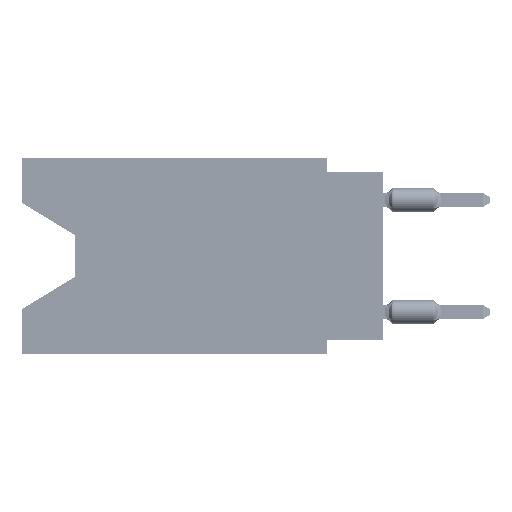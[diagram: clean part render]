
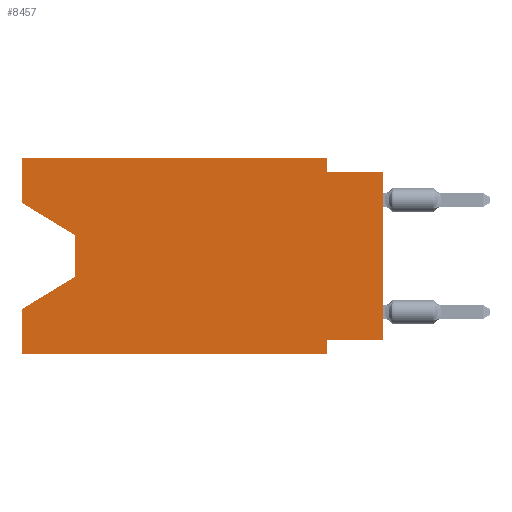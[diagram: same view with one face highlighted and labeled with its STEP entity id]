
A CAD part, left-side view. The second image highlights one B-rep face of the part: STEP entity #8457.
In plain terms, the highlighted planar face has unit normal (-1, 0, 0).
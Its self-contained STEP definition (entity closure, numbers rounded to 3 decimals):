
#1317 = ORIENTED_EDGE ( 'NONE', *, *, #39299, .T. ) ;
#1532 = DIRECTION ( 'NONE',  ( 0., -1., 0. ) ) ;
#1831 = EDGE_CURVE ( 'NONE', #32537, #29362, #54816, .T. ) ;
#2239 = DIRECTION ( 'NONE',  ( 0., 1., 0. ) ) ;
#2278 = LINE ( 'NONE', #7895, #40088 ) ;
#2956 = EDGE_CURVE ( 'NONE', #59551, #34029, #50661, .T. ) ;
#6579 = EDGE_CURVE ( 'NONE', #72040, #9391, #73332, .T. ) ;
#7839 = EDGE_CURVE ( 'NONE', #36415, #64569, #8809, .T. ) ;
#7856 = CARTESIAN_POINT ( 'NONE',  ( 0., 13.97, -3.505 ) ) ;
#7895 = CARTESIAN_POINT ( 'NONE',  ( 0., 0., -0.635 ) ) ;
#8457 = ADVANCED_FACE ( 'NONE', ( #12666 ), #17926, .F. ) ;
#8486 = VECTOR ( 'NONE', #14846, 1000. ) ;
#8809 = LINE ( 'NONE', #20768, #47941 ) ;
#9391 = VERTEX_POINT ( 'NONE', #51396 ) ;
#11251 = CARTESIAN_POINT ( 'NONE',  ( 0., 16.383, -8.89 ) ) ;
#12129 = EDGE_CURVE ( 'NONE', #32537, #13895, #23653, .T. ) ;
#12666 = FACE_OUTER_BOUND ( 'NONE', #43192, .T. ) ;
#13191 = VECTOR ( 'NONE', #67030, 1000. ) ;
#13895 = VERTEX_POINT ( 'NONE', #16146 ) ;
#14657 = CARTESIAN_POINT ( 'NONE',  ( 0., 2.54, 0. ) ) ;
#14846 = DIRECTION ( 'NONE',  ( 0., -1., 0. ) ) ;
#16146 = CARTESIAN_POINT ( 'NONE',  ( 0., 16.383, 0. ) ) ;
#17688 = CARTESIAN_POINT ( 'NONE',  ( 0., 16.383, -6.852 ) ) ;
#17926 = PLANE ( 'NONE',  #39604 ) ;
#19988 = LINE ( 'NONE', #38624, #63804 ) ;
#20069 = DIRECTION ( 'NONE',  ( 0., 0., -1. ) ) ;
#20768 = CARTESIAN_POINT ( 'NONE',  ( 0., 2.54, 0. ) ) ;
#22846 = ORIENTED_EDGE ( 'NONE', *, *, #31156, .F. ) ;
#23537 = CARTESIAN_POINT ( 'NONE',  ( 0., 16.383, 0. ) ) ;
#23653 = LINE ( 'NONE', #34512, #50712 ) ;
#23968 = CARTESIAN_POINT ( 'NONE',  ( 0., 2.54, -0.635 ) ) ;
#25580 = ORIENTED_EDGE ( 'NONE', *, *, #12129, .F. ) ;
#25670 = LINE ( 'NONE', #48467, #49607 ) ;
#26773 = CARTESIAN_POINT ( 'NONE',  ( 0., 16.383, -2.038 ) ) ;
#27480 = DIRECTION ( 'NONE',  ( 0., -1., 0. ) ) ;
#29302 = CARTESIAN_POINT ( 'NONE',  ( 0., 13.97, -5.385 ) ) ;
#29362 = VERTEX_POINT ( 'NONE', #7856 ) ;
#29378 = EDGE_CURVE ( 'NONE', #59551, #72040, #69997, .T. ) ;
#31156 = EDGE_CURVE ( 'NONE', #13895, #36415, #43556, .T. ) ;
#31538 = EDGE_CURVE ( 'NONE', #60661, #9391, #49232, .T. ) ;
#32381 = DIRECTION ( 'NONE',  ( 0., -0.855, -0.519 ) ) ;
#32537 = VERTEX_POINT ( 'NONE', #41522 ) ;
#33281 = CARTESIAN_POINT ( 'NONE',  ( 0., 2.54, -8.89 ) ) ;
#33867 = VECTOR ( 'NONE', #32381, 1000. ) ;
#34029 = VERTEX_POINT ( 'NONE', #59555 ) ;
#34512 = CARTESIAN_POINT ( 'NONE',  ( 0., 16.383, 0. ) ) ;
#36189 = VERTEX_POINT ( 'NONE', #17688 ) ;
#36415 = VERTEX_POINT ( 'NONE', #14657 ) ;
#38321 = DIRECTION ( 'NONE',  ( 0., 0., -1. ) ) ;
#38624 = CARTESIAN_POINT ( 'NONE',  ( 0., 16.383, 0. ) ) ;
#39072 = CARTESIAN_POINT ( 'NONE',  ( 0., 0., 0. ) ) ;
#39299 = EDGE_CURVE ( 'NONE', #67151, #36189, #50138, .T. ) ;
#39604 = AXIS2_PLACEMENT_3D ( 'NONE', #23537, #57204, #45593 ) ;
#40036 = ORIENTED_EDGE ( 'NONE', *, *, #47561, .T. ) ;
#40088 = VECTOR ( 'NONE', #1532, 1000. ) ;
#40442 = VECTOR ( 'NONE', #2239, 1000. ) ;
#41522 = CARTESIAN_POINT ( 'NONE',  ( 0., 16.383, -2.038 ) ) ;
#43192 = EDGE_LOOP ( 'NONE', ( #73643, #40036, #1317, #61124, #62917, #47875, #58562, #63576, #51695, #69534, #22846, #25580 ) ) ;
#43556 = LINE ( 'NONE', #72042, #58555 ) ;
#43893 = DIRECTION ( 'NONE',  ( 0., 0., 1. ) ) ;
#45593 = DIRECTION ( 'NONE',  ( 0., 0., -1. ) ) ;
#46749 = CARTESIAN_POINT ( 'NONE',  ( 0., 0., -8.255 ) ) ;
#47561 = EDGE_CURVE ( 'NONE', #29362, #67151, #25670, .T. ) ;
#47875 = ORIENTED_EDGE ( 'NONE', *, *, #6579, .F. ) ;
#47941 = VECTOR ( 'NONE', #38321, 1000. ) ;
#48467 = CARTESIAN_POINT ( 'NONE',  ( 0., 13.97, -3.505 ) ) ;
#49232 = LINE ( 'NONE', #67580, #8486 ) ;
#49607 = VECTOR ( 'NONE', #20069, 1000. ) ;
#50138 = LINE ( 'NONE', #67762, #13191 ) ;
#50661 = LINE ( 'NONE', #39072, #69682 ) ;
#50712 = VECTOR ( 'NONE', #64442, 1000. ) ;
#50819 = DIRECTION ( 'NONE',  ( 0., 0., -1. ) ) ;
#51396 = CARTESIAN_POINT ( 'NONE',  ( 0., 2.54, -8.89 ) ) ;
#51695 = ORIENTED_EDGE ( 'NONE', *, *, #70637, .F. ) ;
#54816 = LINE ( 'NONE', #26773, #33867 ) ;
#56887 = EDGE_CURVE ( 'NONE', #60661, #36189, #19988, .T. ) ;
#57204 = DIRECTION ( 'NONE',  ( 1., 0., 0. ) ) ;
#58555 = VECTOR ( 'NONE', #27480, 1000. ) ;
#58562 = ORIENTED_EDGE ( 'NONE', *, *, #29378, .F. ) ;
#59551 = VERTEX_POINT ( 'NONE', #46749 ) ;
#59555 = CARTESIAN_POINT ( 'NONE',  ( 0., 0., -0.635 ) ) ;
#60661 = VERTEX_POINT ( 'NONE', #11251 ) ;
#61067 = CARTESIAN_POINT ( 'NONE',  ( 0., 2.54, -8.255 ) ) ;
#61124 = ORIENTED_EDGE ( 'NONE', *, *, #56887, .F. ) ;
#61914 = DIRECTION ( 'NONE',  ( 0., 0., 1. ) ) ;
#62108 = VECTOR ( 'NONE', #50819, 1000. ) ;
#62917 = ORIENTED_EDGE ( 'NONE', *, *, #31538, .T. ) ;
#63576 = ORIENTED_EDGE ( 'NONE', *, *, #2956, .T. ) ;
#63622 = CARTESIAN_POINT ( 'NONE',  ( 0., 0., -8.255 ) ) ;
#63804 = VECTOR ( 'NONE', #43893, 1000. ) ;
#64442 = DIRECTION ( 'NONE',  ( 0., 0., 1. ) ) ;
#64569 = VERTEX_POINT ( 'NONE', #23968 ) ;
#67030 = DIRECTION ( 'NONE',  ( 0., 0.855, -0.519 ) ) ;
#67151 = VERTEX_POINT ( 'NONE', #29302 ) ;
#67580 = CARTESIAN_POINT ( 'NONE',  ( 0., 16.383, -8.89 ) ) ;
#67762 = CARTESIAN_POINT ( 'NONE',  ( 0., 13.97, -5.385 ) ) ;
#69534 = ORIENTED_EDGE ( 'NONE', *, *, #7839, .F. ) ;
#69682 = VECTOR ( 'NONE', #61914, 1000. ) ;
#69997 = LINE ( 'NONE', #63622, #40442 ) ;
#70637 = EDGE_CURVE ( 'NONE', #64569, #34029, #2278, .T. ) ;
#72040 = VERTEX_POINT ( 'NONE', #61067 ) ;
#72042 = CARTESIAN_POINT ( 'NONE',  ( 0., 16.383, 0. ) ) ;
#73332 = LINE ( 'NONE', #33281, #62108 ) ;
#73643 = ORIENTED_EDGE ( 'NONE', *, *, #1831, .T. ) ;
